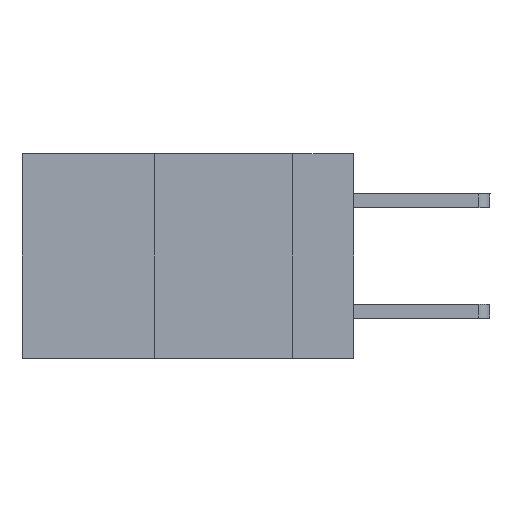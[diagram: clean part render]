
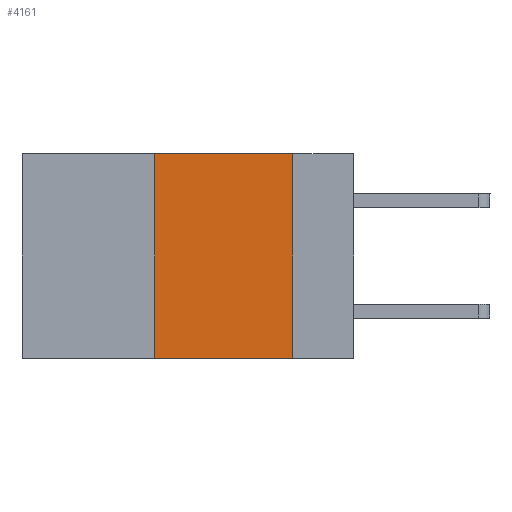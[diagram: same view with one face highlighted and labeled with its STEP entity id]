
A CAD part, left-side view. The second image highlights one B-rep face of the part: STEP entity #4161.
In plain terms, the highlighted planar face has unit normal (-1, 0, 0).
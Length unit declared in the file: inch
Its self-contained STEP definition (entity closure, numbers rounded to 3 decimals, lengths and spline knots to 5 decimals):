
#136 = VECTOR ( 'NONE', #6775, 39.37008 ) ;
#393 = ORIENTED_EDGE ( 'NONE', *, *, #6844, .F. ) ;
#1421 = DIRECTION ( 'NONE',  ( 0., 0., -1. ) ) ;
#1745 = CARTESIAN_POINT ( 'NONE',  ( 0., 0.36, 0. ) ) ;
#2205 = VECTOR ( 'NONE', #5092, 39.37008 ) ;
#2814 = DIRECTION ( 'NONE',  ( 1., 0., 0. ) ) ;
#3272 = CARTESIAN_POINT ( 'NONE',  ( 0., 0.11, 0. ) ) ;
#3314 = EDGE_CURVE ( 'NONE', #6375, #8662, #4531, .T. ) ;
#3912 = EDGE_CURVE ( 'NONE', #4488, #8662, #9740, .T. ) ;
#4133 = CARTESIAN_POINT ( 'NONE',  ( 0., 0.11, -0.37 ) ) ;
#4161 = ADVANCED_FACE ( 'NONE', ( #4669 ), #8431, .F. ) ;
#4488 = VERTEX_POINT ( 'NONE', #10626 ) ;
#4531 = LINE ( 'NONE', #3272, #8705 ) ;
#4669 = FACE_OUTER_BOUND ( 'NONE', #7690, .T. ) ;
#5092 = DIRECTION ( 'NONE',  ( 0., -1., 0. ) ) ;
#5490 = CARTESIAN_POINT ( 'NONE',  ( 0., 0.36, 0. ) ) ;
#5512 = ORIENTED_EDGE ( 'NONE', *, *, #9400, .F. ) ;
#6347 = CARTESIAN_POINT ( 'NONE',  ( 0., 0.11, 0. ) ) ;
#6375 = VERTEX_POINT ( 'NONE', #6347 ) ;
#6775 = DIRECTION ( 'NONE',  ( 0., -1., 0. ) ) ;
#6810 = VECTOR ( 'NONE', #11053, 39.37008 ) ;
#6844 = EDGE_CURVE ( 'NONE', #4488, #11191, #11113, .T. ) ;
#7690 = EDGE_LOOP ( 'NONE', ( #8484, #5512, #393, #10477 ) ) ;
#8431 = PLANE ( 'NONE',  #9131 ) ;
#8472 = CARTESIAN_POINT ( 'NONE',  ( 0., 0.6, 0. ) ) ;
#8484 = ORIENTED_EDGE ( 'NONE', *, *, #3314, .F. ) ;
#8662 = VERTEX_POINT ( 'NONE', #4133 ) ;
#8705 = VECTOR ( 'NONE', #1421, 39.37008 ) ;
#8813 = CARTESIAN_POINT ( 'NONE',  ( 0., 0.6, -0.37 ) ) ;
#9131 = AXIS2_PLACEMENT_3D ( 'NONE', #11285, #2814, #11093 ) ;
#9400 = EDGE_CURVE ( 'NONE', #11191, #6375, #9582, .T. ) ;
#9582 = LINE ( 'NONE', #8472, #136 ) ;
#9740 = LINE ( 'NONE', #8813, #2205 ) ;
#10477 = ORIENTED_EDGE ( 'NONE', *, *, #3912, .T. ) ;
#10626 = CARTESIAN_POINT ( 'NONE',  ( 0., 0.36, -0.37 ) ) ;
#11053 = DIRECTION ( 'NONE',  ( 0., 0., 1. ) ) ;
#11093 = DIRECTION ( 'NONE',  ( 0., 0., -1. ) ) ;
#11113 = LINE ( 'NONE', #5490, #6810 ) ;
#11191 = VERTEX_POINT ( 'NONE', #1745 ) ;
#11285 = CARTESIAN_POINT ( 'NONE',  ( 0., 0.6, 0. ) ) ;
